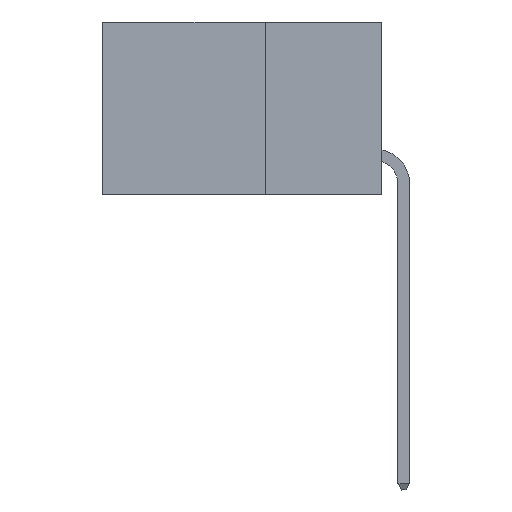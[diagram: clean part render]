
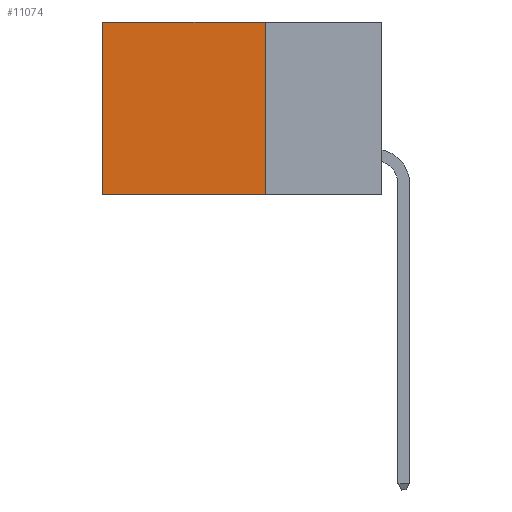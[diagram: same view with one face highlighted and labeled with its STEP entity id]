
A CAD part, left-side view. The second image highlights one B-rep face of the part: STEP entity #11074.
In plain terms, the highlighted planar face has unit normal (-1, 0, 0).
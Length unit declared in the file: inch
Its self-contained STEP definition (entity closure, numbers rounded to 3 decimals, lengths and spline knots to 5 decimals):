
#156 = ORIENTED_EDGE ( 'NONE', *, *, #9212, .T. ) ;
#233 = FACE_OUTER_BOUND ( 'NONE', #12691, .T. ) ;
#303 = DIRECTION ( 'NONE',  ( 1., 0., 0. ) ) ;
#307 = EDGE_CURVE ( 'NONE', #3163, #11905, #7049, .T. ) ;
#1173 = VECTOR ( 'NONE', #2013, 39.37008 ) ;
#1371 = DIRECTION ( 'NONE',  ( 0., 0., -1. ) ) ;
#1884 = CARTESIAN_POINT ( 'NONE',  ( 0.2875, 0.25, -0.37 ) ) ;
#1933 = CARTESIAN_POINT ( 'NONE',  ( 0.2875, 0.25, 0. ) ) ;
#2013 = DIRECTION ( 'NONE',  ( 0., 0., -1. ) ) ;
#2351 = VERTEX_POINT ( 'NONE', #8668 ) ;
#2388 = DIRECTION ( 'NONE',  ( 0., 0., -1. ) ) ;
#2505 = ORIENTED_EDGE ( 'NONE', *, *, #12274, .T. ) ;
#2524 = PLANE ( 'NONE',  #8033 ) ;
#2865 = DIRECTION ( 'NONE',  ( 0., 1., 0. ) ) ;
#3163 = VERTEX_POINT ( 'NONE', #7378 ) ;
#4467 = CARTESIAN_POINT ( 'NONE',  ( 0.2875, 0.25, 0. ) ) ;
#4520 = LINE ( 'NONE', #1933, #1173 ) ;
#6175 = VERTEX_POINT ( 'NONE', #6725 ) ;
#6261 = ORIENTED_EDGE ( 'NONE', *, *, #12746, .F. ) ;
#6415 = CARTESIAN_POINT ( 'NONE',  ( 0.2875, 0.6, 0. ) ) ;
#6725 = CARTESIAN_POINT ( 'NONE',  ( 0.2875, 0.6, 0. ) ) ;
#7049 = LINE ( 'NONE', #1884, #10074 ) ;
#7378 = CARTESIAN_POINT ( 'NONE',  ( 0.2875, 0.25, -0.37 ) ) ;
#7683 = VECTOR ( 'NONE', #1371, 39.37008 ) ;
#7859 = CARTESIAN_POINT ( 'NONE',  ( 0.2875, 0.25, 0. ) ) ;
#8033 = AXIS2_PLACEMENT_3D ( 'NONE', #4467, #303, #2388 ) ;
#8668 = CARTESIAN_POINT ( 'NONE',  ( 0.2875, 0.25, 0. ) ) ;
#8804 = DIRECTION ( 'NONE',  ( 0., 1., 0. ) ) ;
#9212 = EDGE_CURVE ( 'NONE', #2351, #6175, #10567, .T. ) ;
#10074 = VECTOR ( 'NONE', #8804, 39.37008 ) ;
#10567 = LINE ( 'NONE', #7859, #10887 ) ;
#10887 = VECTOR ( 'NONE', #2865, 39.37008 ) ;
#11074 = ADVANCED_FACE ( 'NONE', ( #233 ), #2524, .F. ) ;
#11227 = ORIENTED_EDGE ( 'NONE', *, *, #307, .F. ) ;
#11905 = VERTEX_POINT ( 'NONE', #11911 ) ;
#11911 = CARTESIAN_POINT ( 'NONE',  ( 0.2875, 0.6, -0.37 ) ) ;
#11956 = LINE ( 'NONE', #6415, #7683 ) ;
#12274 = EDGE_CURVE ( 'NONE', #6175, #11905, #11956, .T. ) ;
#12691 = EDGE_LOOP ( 'NONE', ( #2505, #11227, #6261, #156 ) ) ;
#12746 = EDGE_CURVE ( 'NONE', #2351, #3163, #4520, .T. ) ;
